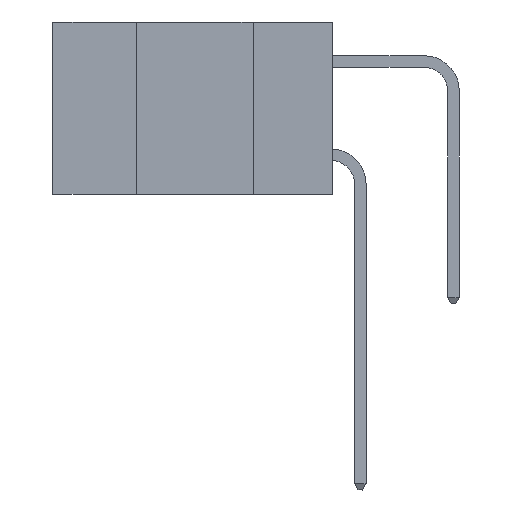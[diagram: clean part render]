
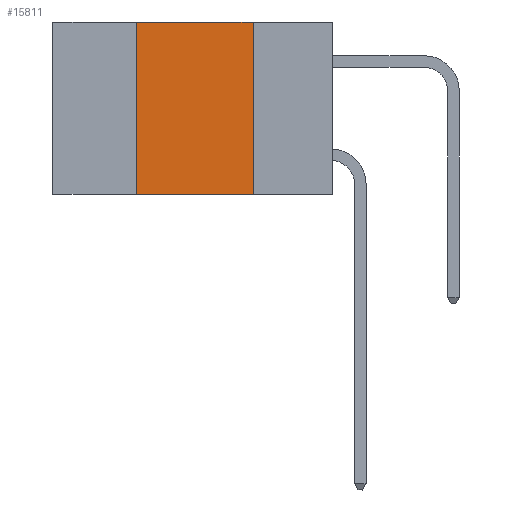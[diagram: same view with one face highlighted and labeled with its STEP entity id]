
A CAD part, left-side view. The second image highlights one B-rep face of the part: STEP entity #15811.
In plain terms, the highlighted planar face has unit normal (-1, 0, 0).
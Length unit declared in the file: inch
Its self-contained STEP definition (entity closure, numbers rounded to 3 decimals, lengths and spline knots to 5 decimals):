
#54 = EDGE_CURVE ( 'NONE', #13477, #21599, #21120, .T. ) ;
#70 = ORIENTED_EDGE ( 'NONE', *, *, #5880, .T. ) ;
#603 = PLANE ( 'NONE',  #1740 ) ;
#1492 = FACE_OUTER_BOUND ( 'NONE', #23316, .T. ) ;
#1576 = LINE ( 'NONE', #16961, #7306 ) ;
#1740 = AXIS2_PLACEMENT_3D ( 'NONE', #9120, #21886, #9215 ) ;
#2075 = DIRECTION ( 'NONE',  ( 0., -1., 0. ) ) ;
#3072 = LINE ( 'NONE', #22254, #13678 ) ;
#4493 = ORIENTED_EDGE ( 'NONE', *, *, #26108, .F. ) ;
#5608 = VERTEX_POINT ( 'NONE', #21562 ) ;
#5880 = EDGE_CURVE ( 'NONE', #5608, #21599, #3072, .T. ) ;
#6637 = DIRECTION ( 'NONE',  ( 0., 0., -1. ) ) ;
#7306 = VECTOR ( 'NONE', #2075, 39.37008 ) ;
#8204 = LINE ( 'NONE', #14010, #18772 ) ;
#9012 = CARTESIAN_POINT ( 'NONE',  ( 0., 0.17, 0. ) ) ;
#9120 = CARTESIAN_POINT ( 'NONE',  ( 0., 0.6, 0. ) ) ;
#9215 = DIRECTION ( 'NONE',  ( 0., 0., -1. ) ) ;
#11736 = CARTESIAN_POINT ( 'NONE',  ( 0., 0.42, 0. ) ) ;
#13477 = VERTEX_POINT ( 'NONE', #9012 ) ;
#13678 = VECTOR ( 'NONE', #13865, 39.37008 ) ;
#13865 = DIRECTION ( 'NONE',  ( 0., -1., 0. ) ) ;
#14010 = CARTESIAN_POINT ( 'NONE',  ( 0., 0.42, 0. ) ) ;
#14113 = DIRECTION ( 'NONE',  ( 0., 0., 1. ) ) ;
#14528 = EDGE_CURVE ( 'NONE', #24789, #13477, #1576, .T. ) ;
#15811 = ADVANCED_FACE ( 'NONE', ( #1492 ), #603, .F. ) ;
#16961 = CARTESIAN_POINT ( 'NONE',  ( 0., 0.6, 0. ) ) ;
#18772 = VECTOR ( 'NONE', #14113, 39.37008 ) ;
#20379 = CARTESIAN_POINT ( 'NONE',  ( 0., 0.17, -0.37 ) ) ;
#20610 = VECTOR ( 'NONE', #6637, 39.37008 ) ;
#20706 = ORIENTED_EDGE ( 'NONE', *, *, #14528, .F. ) ;
#21120 = LINE ( 'NONE', #21638, #20610 ) ;
#21562 = CARTESIAN_POINT ( 'NONE',  ( 0., 0.42, -0.37 ) ) ;
#21599 = VERTEX_POINT ( 'NONE', #20379 ) ;
#21638 = CARTESIAN_POINT ( 'NONE',  ( 0., 0.17, 0. ) ) ;
#21886 = DIRECTION ( 'NONE',  ( 1., 0., 0. ) ) ;
#22254 = CARTESIAN_POINT ( 'NONE',  ( 0., 0.6, -0.37 ) ) ;
#23316 = EDGE_LOOP ( 'NONE', ( #25561, #20706, #4493, #70 ) ) ;
#24789 = VERTEX_POINT ( 'NONE', #11736 ) ;
#25561 = ORIENTED_EDGE ( 'NONE', *, *, #54, .F. ) ;
#26108 = EDGE_CURVE ( 'NONE', #5608, #24789, #8204, .T. ) ;
